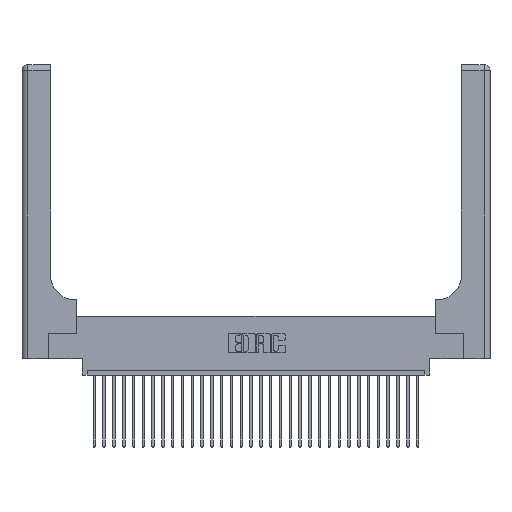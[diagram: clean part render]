
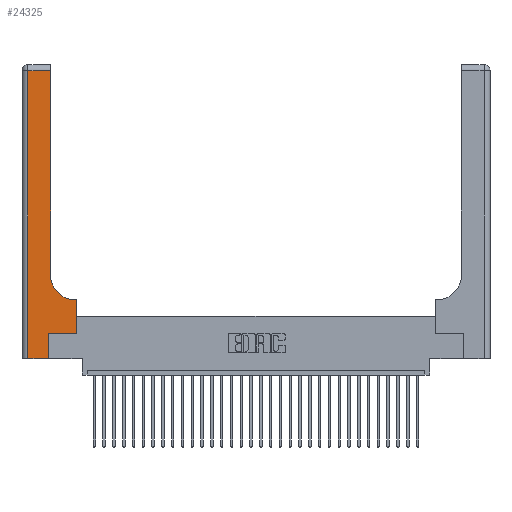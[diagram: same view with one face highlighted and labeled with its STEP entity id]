
A CAD part, top view. The second image highlights one B-rep face of the part: STEP entity #24325.
In plain terms, the highlighted planar face has unit normal (0, 0, 1).
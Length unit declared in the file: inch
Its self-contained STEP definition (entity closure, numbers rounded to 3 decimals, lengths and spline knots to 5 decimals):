
#701 = DIRECTION ( 'NONE',  ( 1., 0., 0. ) ) ;
#3471 = LINE ( 'NONE', #21968, #28136 ) ;
#4565 = EDGE_CURVE ( 'NONE', #31567, #22138, #30622, .T. ) ;
#4735 = LINE ( 'NONE', #16936, #27833 ) ;
#5453 = CARTESIAN_POINT ( 'NONE',  ( 0.269, 0.25, 0.37 ) ) ;
#5749 = ORIENTED_EDGE ( 'NONE', *, *, #24295, .T. ) ;
#6209 = ORIENTED_EDGE ( 'NONE', *, *, #7187, .T. ) ;
#6954 = ORIENTED_EDGE ( 'NONE', *, *, #20001, .T. ) ;
#7187 = EDGE_CURVE ( 'NONE', #28794, #27481, #26584, .T. ) ;
#8275 = CARTESIAN_POINT ( 'NONE',  ( 0.5415, 0.85, 0.37 ) ) ;
#8278 = ORIENTED_EDGE ( 'NONE', *, *, #18885, .T. ) ;
#8468 = CARTESIAN_POINT ( 'NONE',  ( 0.06, 3., 0.37 ) ) ;
#8674 = CARTESIAN_POINT ( 'NONE',  ( 0., 3., 0.37 ) ) ;
#9603 = DIRECTION ( 'NONE',  ( 1., 0., 0. ) ) ;
#9933 = LINE ( 'NONE', #11648, #29573 ) ;
#10594 = EDGE_LOOP ( 'NONE', ( #6209, #20013, #5749, #25915, #28970, #8278, #26765, #6954, #29585 ) ) ;
#11161 = DIRECTION ( 'NONE',  ( 0., -1., 0. ) ) ;
#11614 = VERTEX_POINT ( 'NONE', #30534 ) ;
#11648 = CARTESIAN_POINT ( 'NONE',  ( 0.269, 0.25, 0.37 ) ) ;
#11675 = DIRECTION ( 'NONE',  ( -1., 0., 0. ) ) ;
#11860 = DIRECTION ( 'NONE',  ( 1., 0., 0. ) ) ;
#12706 = CARTESIAN_POINT ( 'NONE',  ( 0.5415, 0.6, 0.37 ) ) ;
#12794 = EDGE_CURVE ( 'NONE', #22920, #29697, #3471, .T. ) ;
#13335 = DIRECTION ( 'NONE',  ( -1., 0., 0. ) ) ;
#13801 = CARTESIAN_POINT ( 'NONE',  ( 0.5585, 0.25, 0.37 ) ) ;
#13830 = CARTESIAN_POINT ( 'NONE',  ( 0., 2.94, 0.37 ) ) ;
#13882 = FACE_OUTER_BOUND ( 'NONE', #10594, .T. ) ;
#15042 = EDGE_CURVE ( 'NONE', #11614, #31567, #4735, .T. ) ;
#16536 = CARTESIAN_POINT ( 'NONE',  ( 0.06, 2.94, 0.37 ) ) ;
#16936 = CARTESIAN_POINT ( 'NONE',  ( 0., 0., 0.37 ) ) ;
#17065 = LINE ( 'NONE', #13830, #26669 ) ;
#17623 = CARTESIAN_POINT ( 'NONE',  ( 0.2915, 0.85, 0.37 ) ) ;
#18582 = DIRECTION ( 'NONE',  ( 0., 0., -1. ) ) ;
#18736 = LINE ( 'NONE', #21330, #27953 ) ;
#18812 = DIRECTION ( 'NONE',  ( 0., 1., 0. ) ) ;
#18885 = EDGE_CURVE ( 'NONE', #22138, #22920, #9933, .T. ) ;
#20001 = EDGE_CURVE ( 'NONE', #29697, #29323, #18736, .T. ) ;
#20013 = ORIENTED_EDGE ( 'NONE', *, *, #30233, .T. ) ;
#20046 = VECTOR ( 'NONE', #18812, 39.37008 ) ;
#20425 = VECTOR ( 'NONE', #11161, 39.37008 ) ;
#20456 = CIRCLE ( 'NONE', #26912, 0.25 ) ;
#20458 = DIRECTION ( 'NONE',  ( 0., 0., -1. ) ) ;
#21330 = CARTESIAN_POINT ( 'NONE',  ( 0.2915, 0.6, 0.37 ) ) ;
#21824 = DIRECTION ( 'NONE',  ( 0., 1., 0. ) ) ;
#21968 = CARTESIAN_POINT ( 'NONE',  ( 0.5585, 0.25, 0.37 ) ) ;
#22138 = VERTEX_POINT ( 'NONE', #5453 ) ;
#22324 = VERTEX_POINT ( 'NONE', #16536 ) ;
#22920 = VERTEX_POINT ( 'NONE', #13801 ) ;
#23598 = EDGE_CURVE ( 'NONE', #29323, #28794, #20456, .T. ) ;
#24295 = EDGE_CURVE ( 'NONE', #22324, #11614, #27723, .T. ) ;
#24325 = ADVANCED_FACE ( 'NONE', ( #13882 ), #28145, .F. ) ;
#24429 = DIRECTION ( 'NONE',  ( 0., 1., 0. ) ) ;
#25900 = CARTESIAN_POINT ( 'NONE',  ( 0.2915, 3., 0.37 ) ) ;
#25915 = ORIENTED_EDGE ( 'NONE', *, *, #15042, .T. ) ;
#26325 = CARTESIAN_POINT ( 'NONE',  ( 0.269, 0., 0.37 ) ) ;
#26584 = LINE ( 'NONE', #25900, #20046 ) ;
#26669 = VECTOR ( 'NONE', #31388, 39.37008 ) ;
#26765 = ORIENTED_EDGE ( 'NONE', *, *, #12794, .T. ) ;
#26912 = AXIS2_PLACEMENT_3D ( 'NONE', #8275, #20458, #701 ) ;
#27481 = VERTEX_POINT ( 'NONE', #27888 ) ;
#27723 = LINE ( 'NONE', #8468, #20425 ) ;
#27833 = VECTOR ( 'NONE', #9603, 39.37008 ) ;
#27888 = CARTESIAN_POINT ( 'NONE',  ( 0.2915, 2.94, 0.37 ) ) ;
#27907 = VECTOR ( 'NONE', #21824, 39.37008 ) ;
#27953 = VECTOR ( 'NONE', #11675, 39.37008 ) ;
#28136 = VECTOR ( 'NONE', #24429, 39.37008 ) ;
#28145 = PLANE ( 'NONE',  #28988 ) ;
#28794 = VERTEX_POINT ( 'NONE', #17623 ) ;
#28970 = ORIENTED_EDGE ( 'NONE', *, *, #4565, .T. ) ;
#28988 = AXIS2_PLACEMENT_3D ( 'NONE', #8674, #18582, #13335 ) ;
#29323 = VERTEX_POINT ( 'NONE', #12706 ) ;
#29573 = VECTOR ( 'NONE', #11860, 39.37008 ) ;
#29585 = ORIENTED_EDGE ( 'NONE', *, *, #23598, .T. ) ;
#29697 = VERTEX_POINT ( 'NONE', #31298 ) ;
#30233 = EDGE_CURVE ( 'NONE', #27481, #22324, #17065, .T. ) ;
#30534 = CARTESIAN_POINT ( 'NONE',  ( 0.06, 0., 0.37 ) ) ;
#30622 = LINE ( 'NONE', #26325, #27907 ) ;
#31298 = CARTESIAN_POINT ( 'NONE',  ( 0.5585, 0.6, 0.37 ) ) ;
#31388 = DIRECTION ( 'NONE',  ( -1., 0., 0. ) ) ;
#31567 = VERTEX_POINT ( 'NONE', #31630 ) ;
#31630 = CARTESIAN_POINT ( 'NONE',  ( 0.269, 0., 0.37 ) ) ;
